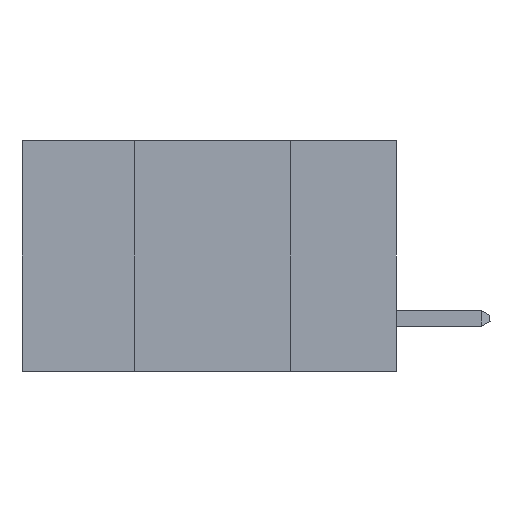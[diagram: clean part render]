
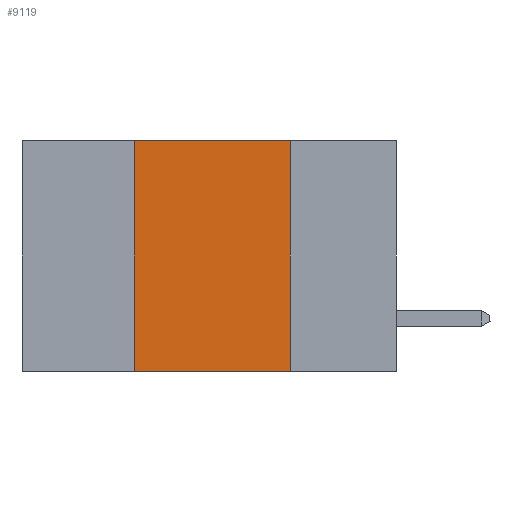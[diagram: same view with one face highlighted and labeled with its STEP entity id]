
A CAD part, left-side view. The second image highlights one B-rep face of the part: STEP entity #9119.
In plain terms, the highlighted planar face has unit normal (-1, 0, 0).
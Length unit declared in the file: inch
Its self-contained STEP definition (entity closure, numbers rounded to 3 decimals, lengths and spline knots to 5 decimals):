
#1259 = DIRECTION ( 'NONE',  ( 0., 0., 1. ) ) ;
#1387 = FACE_OUTER_BOUND ( 'NONE', #11896, .T. ) ;
#2630 = LINE ( 'NONE', #6655, #17120 ) ;
#2994 = DIRECTION ( 'NONE',  ( 1., 0., 0. ) ) ;
#3374 = ORIENTED_EDGE ( 'NONE', *, *, #5264, .F. ) ;
#4222 = DIRECTION ( 'NONE',  ( 0., -1., 0. ) ) ;
#4312 = CARTESIAN_POINT ( 'NONE',  ( 0., 0.42, -0.37 ) ) ;
#4429 = VECTOR ( 'NONE', #4222, 39.37008 ) ;
#5259 = VERTEX_POINT ( 'NONE', #11919 ) ;
#5264 = EDGE_CURVE ( 'NONE', #18038, #17849, #6764, .T. ) ;
#5584 = VECTOR ( 'NONE', #9982, 39.37008 ) ;
#6423 = ORIENTED_EDGE ( 'NONE', *, *, #19136, .F. ) ;
#6595 = ORIENTED_EDGE ( 'NONE', *, *, #14301, .F. ) ;
#6655 = CARTESIAN_POINT ( 'NONE',  ( 0., 0.17, 0. ) ) ;
#6764 = LINE ( 'NONE', #22177, #5584 ) ;
#9119 = ADVANCED_FACE ( 'NONE', ( #1387 ), #20989, .F. ) ;
#9982 = DIRECTION ( 'NONE',  ( 0., -1., 0. ) ) ;
#11896 = EDGE_LOOP ( 'NONE', ( #6423, #3374, #6595, #19073 ) ) ;
#11919 = CARTESIAN_POINT ( 'NONE',  ( 0., 0.17, -0.37 ) ) ;
#13546 = LINE ( 'NONE', #16913, #4429 ) ;
#13881 = CARTESIAN_POINT ( 'NONE',  ( 0., 0.6, 0. ) ) ;
#14301 = EDGE_CURVE ( 'NONE', #20116, #18038, #19464, .T. ) ;
#15668 = DIRECTION ( 'NONE',  ( 0., 0., -1. ) ) ;
#16913 = CARTESIAN_POINT ( 'NONE',  ( 0., 0.6, -0.37 ) ) ;
#17120 = VECTOR ( 'NONE', #19221, 39.37008 ) ;
#17849 = VERTEX_POINT ( 'NONE', #21420 ) ;
#18019 = AXIS2_PLACEMENT_3D ( 'NONE', #13881, #2994, #15668 ) ;
#18038 = VERTEX_POINT ( 'NONE', #21956 ) ;
#18696 = EDGE_CURVE ( 'NONE', #20116, #5259, #13546, .T. ) ;
#19073 = ORIENTED_EDGE ( 'NONE', *, *, #18696, .T. ) ;
#19136 = EDGE_CURVE ( 'NONE', #17849, #5259, #2630, .T. ) ;
#19221 = DIRECTION ( 'NONE',  ( 0., 0., -1. ) ) ;
#19464 = LINE ( 'NONE', #22862, #23041 ) ;
#20116 = VERTEX_POINT ( 'NONE', #4312 ) ;
#20989 = PLANE ( 'NONE',  #18019 ) ;
#21420 = CARTESIAN_POINT ( 'NONE',  ( 0., 0.17, 0. ) ) ;
#21956 = CARTESIAN_POINT ( 'NONE',  ( 0., 0.42, 0. ) ) ;
#22177 = CARTESIAN_POINT ( 'NONE',  ( 0., 0.6, 0. ) ) ;
#22862 = CARTESIAN_POINT ( 'NONE',  ( 0., 0.42, 0. ) ) ;
#23041 = VECTOR ( 'NONE', #1259, 39.37008 ) ;
